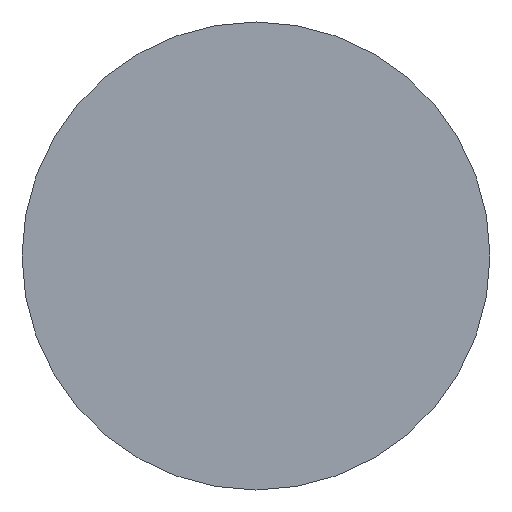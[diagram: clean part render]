
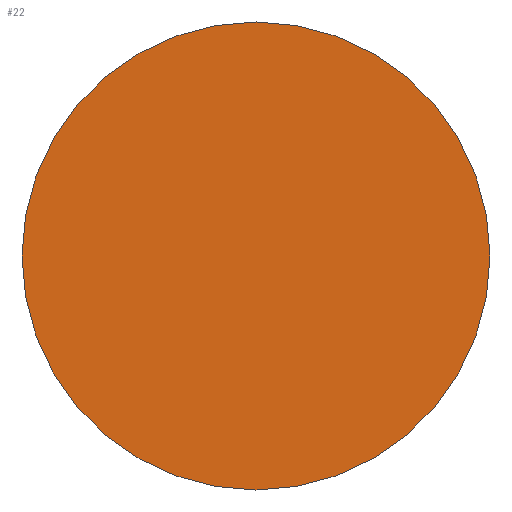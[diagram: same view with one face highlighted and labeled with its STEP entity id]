
A CAD part, left-side view. The second image highlights one B-rep face of the part: STEP entity #22.
In plain terms, the highlighted planar face has unit normal (-1, 0, 0).
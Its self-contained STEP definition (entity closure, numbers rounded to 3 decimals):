
#8 = ORIENTED_EDGE ( 'NONE', *, *, #87, .F. ) ;
#10 = DIRECTION ( 'NONE',  ( -1., 0., 0. ) ) ;
#13 = DIRECTION ( 'NONE',  ( 0., 0., 1. ) ) ;
#22 = ADVANCED_FACE ( 'NONE', ( #162 ), #172, .T. ) ;
#28 = CARTESIAN_POINT ( 'NONE',  ( -194.682, 23.547, -5.019 ) ) ;
#30 = VERTEX_POINT ( 'NONE', #160 ) ;
#36 = CIRCLE ( 'NONE', #78, 2. ) ;
#62 = DIRECTION ( 'NONE',  ( 0., 0., 1. ) ) ;
#64 = DIRECTION ( 'NONE',  ( 1., 0., 0. ) ) ;
#69 = CIRCLE ( 'NONE', #99, 2. ) ;
#70 = VERTEX_POINT ( 'NONE', #73 ) ;
#72 = AXIS2_PLACEMENT_3D ( 'NONE', #28, #10, #13 ) ;
#73 = CARTESIAN_POINT ( 'NONE',  ( -194.682, 23.547, -7.019 ) ) ;
#78 = AXIS2_PLACEMENT_3D ( 'NONE', #84, #104, #159 ) ;
#84 = CARTESIAN_POINT ( 'NONE',  ( -194.682, 23.547, -5.019 ) ) ;
#87 = EDGE_CURVE ( 'NONE', #70, #30, #36, .T. ) ;
#99 = AXIS2_PLACEMENT_3D ( 'NONE', #168, #64, #62 ) ;
#100 = EDGE_LOOP ( 'NONE', ( #120, #8 ) ) ;
#104 = DIRECTION ( 'NONE',  ( 1., 0., 0. ) ) ;
#120 = ORIENTED_EDGE ( 'NONE', *, *, #144, .F. ) ;
#144 = EDGE_CURVE ( 'NONE', #30, #70, #69, .T. ) ;
#159 = DIRECTION ( 'NONE',  ( 0., 0., 1. ) ) ;
#160 = CARTESIAN_POINT ( 'NONE',  ( -194.682, 23.547, -3.019 ) ) ;
#162 = FACE_OUTER_BOUND ( 'NONE', #100, .T. ) ;
#168 = CARTESIAN_POINT ( 'NONE',  ( -194.682, 23.547, -5.019 ) ) ;
#172 = PLANE ( 'NONE',  #72 ) ;
